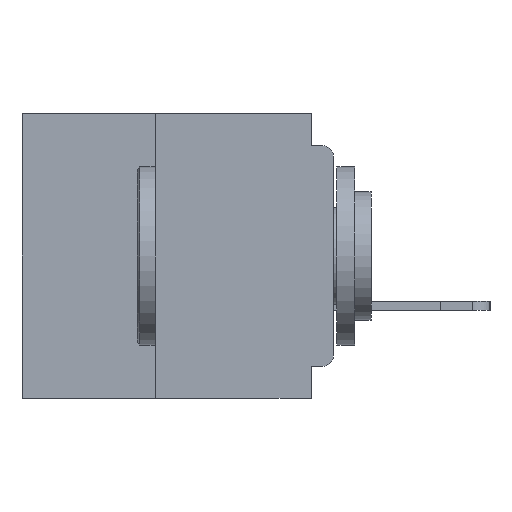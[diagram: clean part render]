
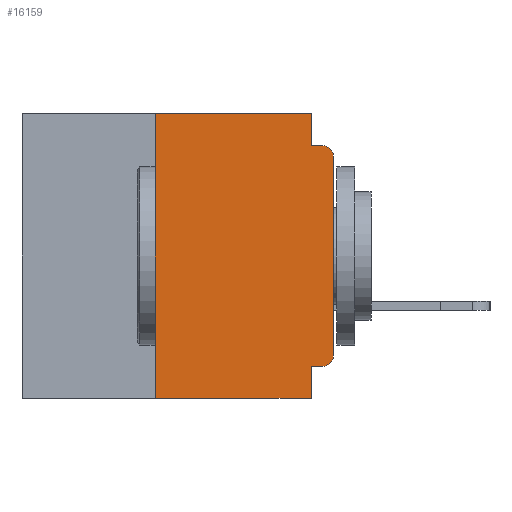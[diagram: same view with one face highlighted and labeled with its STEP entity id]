
A CAD part, left-side view. The second image highlights one B-rep face of the part: STEP entity #16159.
In plain terms, the highlighted planar face has unit normal (-1, 0, 0).
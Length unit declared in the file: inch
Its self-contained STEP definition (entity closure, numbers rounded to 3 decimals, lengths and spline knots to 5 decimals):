
#448 = CARTESIAN_POINT ( 'NONE',  ( 0., 0., -0.355 ) ) ;
#505 = VERTEX_POINT ( 'NONE', #3884 ) ;
#886 = LINE ( 'NONE', #1536, #36939 ) ;
#1447 = DIRECTION ( 'NONE',  ( 0., -1., 0. ) ) ;
#1536 = CARTESIAN_POINT ( 'NONE',  ( 0., 0.437, -0.4 ) ) ;
#2212 = VERTEX_POINT ( 'NONE', #21741 ) ;
#3422 = CARTESIAN_POINT ( 'NONE',  ( 0., 0.031, -0.355 ) ) ;
#3884 = CARTESIAN_POINT ( 'NONE',  ( 0., 0.031, -0.045 ) ) ;
#4176 = AXIS2_PLACEMENT_3D ( 'NONE', #8221, #32644, #11722 ) ;
#5090 = VECTOR ( 'NONE', #10857, 39.37008 ) ;
#5467 = EDGE_CURVE ( 'NONE', #12324, #17618, #886, .T. ) ;
#5789 = EDGE_CURVE ( 'NONE', #505, #13513, #37750, .T. ) ;
#6127 = CARTESIAN_POINT ( 'NONE',  ( 0., 0.437, 0. ) ) ;
#6167 = CARTESIAN_POINT ( 'NONE',  ( 0., 0.015, -0.355 ) ) ;
#6522 = CARTESIAN_POINT ( 'NONE',  ( 0., 0.25, -0.4 ) ) ;
#6793 = VECTOR ( 'NONE', #23512, 39.37008 ) ;
#8221 = CARTESIAN_POINT ( 'NONE',  ( 0., 0.437, 0. ) ) ;
#8725 = CIRCLE ( 'NONE', #32899, 0.015 ) ;
#9105 = ORIENTED_EDGE ( 'NONE', *, *, #9502, .T. ) ;
#9502 = EDGE_CURVE ( 'NONE', #38814, #29427, #30385, .T. ) ;
#9743 = LINE ( 'NONE', #37739, #11896 ) ;
#9751 = DIRECTION ( 'NONE',  ( -1., 0., 0. ) ) ;
#10857 = DIRECTION ( 'NONE',  ( 0., 1., 0. ) ) ;
#11722 = DIRECTION ( 'NONE',  ( 0., 0., -1. ) ) ;
#11896 = VECTOR ( 'NONE', #34240, 39.37008 ) ;
#12297 = ORIENTED_EDGE ( 'NONE', *, *, #5467, .T. ) ;
#12324 = VERTEX_POINT ( 'NONE', #6522 ) ;
#12840 = ORIENTED_EDGE ( 'NONE', *, *, #28173, .F. ) ;
#13513 = VERTEX_POINT ( 'NONE', #30550 ) ;
#14425 = DIRECTION ( 'NONE',  ( -1., 0., 0. ) ) ;
#15035 = CARTESIAN_POINT ( 'NONE',  ( 0., 0., -0.34 ) ) ;
#16159 = ADVANCED_FACE ( 'NONE', ( #32759 ), #39512, .F. ) ;
#16812 = CARTESIAN_POINT ( 'NONE',  ( 0., 0.031, -0.4 ) ) ;
#17133 = EDGE_CURVE ( 'NONE', #12324, #2212, #9743, .T. ) ;
#17324 = EDGE_LOOP ( 'NONE', ( #22858, #41677, #19839, #21879, #39806, #34565, #12297, #12840, #21908, #9105 ) ) ;
#17618 = VERTEX_POINT ( 'NONE', #40472 ) ;
#18229 = LINE ( 'NONE', #6127, #6793 ) ;
#19839 = ORIENTED_EDGE ( 'NONE', *, *, #5789, .F. ) ;
#19843 = VERTEX_POINT ( 'NONE', #3422 ) ;
#20324 = DIRECTION ( 'NONE',  ( 0., 0., -1. ) ) ;
#21268 = VECTOR ( 'NONE', #20324, 39.37008 ) ;
#21741 = CARTESIAN_POINT ( 'NONE',  ( 0., 0.25, 0. ) ) ;
#21879 = ORIENTED_EDGE ( 'NONE', *, *, #36170, .F. ) ;
#21908 = ORIENTED_EDGE ( 'NONE', *, *, #22201, .F. ) ;
#21985 = EDGE_CURVE ( 'NONE', #2212, #23336, #18229, .T. ) ;
#22201 = EDGE_CURVE ( 'NONE', #38814, #19843, #32968, .T. ) ;
#22858 = ORIENTED_EDGE ( 'NONE', *, *, #25703, .T. ) ;
#23336 = VERTEX_POINT ( 'NONE', #45260 ) ;
#23512 = DIRECTION ( 'NONE',  ( 0., -1., 0. ) ) ;
#25703 = EDGE_CURVE ( 'NONE', #29427, #43556, #35704, .T. ) ;
#27641 = DIRECTION ( 'NONE',  ( 0., 0., 1. ) ) ;
#28136 = DIRECTION ( 'NONE',  ( 0., 0., -1. ) ) ;
#28173 = EDGE_CURVE ( 'NONE', #19843, #17618, #30560, .T. ) ;
#29427 = VERTEX_POINT ( 'NONE', #15035 ) ;
#29568 = VECTOR ( 'NONE', #33303, 39.37008 ) ;
#30385 = CIRCLE ( 'NONE', #32452, 0.015 ) ;
#30550 = CARTESIAN_POINT ( 'NONE',  ( 0., 0.015, -0.045 ) ) ;
#30560 = LINE ( 'NONE', #16812, #21268 ) ;
#30661 = CARTESIAN_POINT ( 'NONE',  ( 0., 0.015, -0.06 ) ) ;
#31422 = CARTESIAN_POINT ( 'NONE',  ( 0., 0., -0.06 ) ) ;
#31609 = VECTOR ( 'NONE', #28136, 39.37008 ) ;
#32452 = AXIS2_PLACEMENT_3D ( 'NONE', #35306, #14425, #38803 ) ;
#32644 = DIRECTION ( 'NONE',  ( 1., 0., 0. ) ) ;
#32759 = FACE_OUTER_BOUND ( 'NONE', #17324, .T. ) ;
#32899 = AXIS2_PLACEMENT_3D ( 'NONE', #30661, #9751, #34144 ) ;
#32968 = LINE ( 'NONE', #448, #5090 ) ;
#33156 = CARTESIAN_POINT ( 'NONE',  ( 0., 0., -0.045 ) ) ;
#33303 = DIRECTION ( 'NONE',  ( 0., -1., 0. ) ) ;
#34144 = DIRECTION ( 'NONE',  ( 0., 0., -1. ) ) ;
#34240 = DIRECTION ( 'NONE',  ( 0., 0., 1. ) ) ;
#34565 = ORIENTED_EDGE ( 'NONE', *, *, #17133, .F. ) ;
#34614 = VECTOR ( 'NONE', #27641, 39.37008 ) ;
#34905 = EDGE_CURVE ( 'NONE', #43556, #13513, #8725, .T. ) ;
#35306 = CARTESIAN_POINT ( 'NONE',  ( 0., 0.015, -0.34 ) ) ;
#35704 = LINE ( 'NONE', #45062, #34614 ) ;
#36170 = EDGE_CURVE ( 'NONE', #23336, #505, #40903, .T. ) ;
#36939 = VECTOR ( 'NONE', #1447, 39.37008 ) ;
#37739 = CARTESIAN_POINT ( 'NONE',  ( 0., 0.25, -0.4 ) ) ;
#37750 = LINE ( 'NONE', #33156, #29568 ) ;
#38803 = DIRECTION ( 'NONE',  ( 0., 0., -1. ) ) ;
#38814 = VERTEX_POINT ( 'NONE', #6167 ) ;
#39512 = PLANE ( 'NONE',  #4176 ) ;
#39806 = ORIENTED_EDGE ( 'NONE', *, *, #21985, .F. ) ;
#40472 = CARTESIAN_POINT ( 'NONE',  ( 0., 0.031, -0.4 ) ) ;
#40903 = LINE ( 'NONE', #42016, #31609 ) ;
#41677 = ORIENTED_EDGE ( 'NONE', *, *, #34905, .T. ) ;
#42016 = CARTESIAN_POINT ( 'NONE',  ( 0., 0.031, 0. ) ) ;
#43556 = VERTEX_POINT ( 'NONE', #31422 ) ;
#45062 = CARTESIAN_POINT ( 'NONE',  ( 0., 0., 0. ) ) ;
#45260 = CARTESIAN_POINT ( 'NONE',  ( 0., 0.031, 0. ) ) ;
